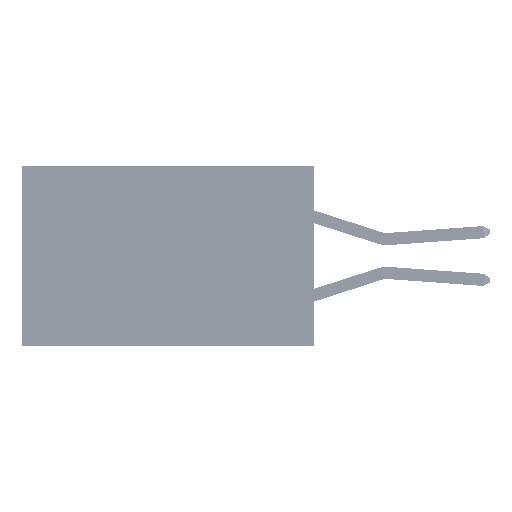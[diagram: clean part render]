
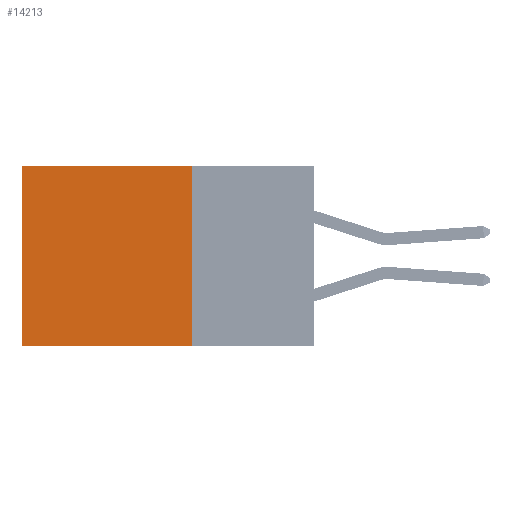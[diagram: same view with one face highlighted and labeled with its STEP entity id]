
A CAD part, left-side view. The second image highlights one B-rep face of the part: STEP entity #14213.
In plain terms, the highlighted planar face has unit normal (-1, 0, 0).
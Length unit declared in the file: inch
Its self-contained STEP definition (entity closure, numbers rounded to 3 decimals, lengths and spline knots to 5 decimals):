
#1226 = VERTEX_POINT ( 'NONE', #41984 ) ;
#1234 = CARTESIAN_POINT ( 'NONE',  ( 0.2875, 0.6, 0. ) ) ;
#1390 = DIRECTION ( 'NONE',  ( 0., 0., -1. ) ) ;
#2283 = EDGE_CURVE ( 'NONE', #33521, #27277, #3901, .T. ) ;
#3901 = LINE ( 'NONE', #34683, #35376 ) ;
#7206 = DIRECTION ( 'NONE',  ( 0., 0., -1. ) ) ;
#7825 = LINE ( 'NONE', #43653, #44966 ) ;
#9397 = DIRECTION ( 'NONE',  ( 0., 1., 0. ) ) ;
#10475 = ORIENTED_EDGE ( 'NONE', *, *, #2283, .F. ) ;
#13474 = VECTOR ( 'NONE', #43438, 39.37008 ) ;
#13929 = DIRECTION ( 'NONE',  ( 1., 0., 0. ) ) ;
#14095 = PLANE ( 'NONE',  #30364 ) ;
#14213 = ADVANCED_FACE ( 'NONE', ( #26748 ), #14095, .F. ) ;
#14412 = VERTEX_POINT ( 'NONE', #1234 ) ;
#14623 = DIRECTION ( 'NONE',  ( 0., 0., -1. ) ) ;
#15392 = VECTOR ( 'NONE', #9397, 39.37008 ) ;
#16209 = EDGE_LOOP ( 'NONE', ( #30724, #36020, #10475, #21837 ) ) ;
#17731 = CARTESIAN_POINT ( 'NONE',  ( 0.2875, 0.25, -0.37 ) ) ;
#20446 = CARTESIAN_POINT ( 'NONE',  ( 0.2875, 0.25, 0. ) ) ;
#21837 = ORIENTED_EDGE ( 'NONE', *, *, #45774, .T. ) ;
#22580 = CARTESIAN_POINT ( 'NONE',  ( 0.2875, 0.25, -0.37 ) ) ;
#23207 = LINE ( 'NONE', #17731, #13474 ) ;
#25975 = EDGE_CURVE ( 'NONE', #27277, #1226, #23207, .T. ) ;
#26748 = FACE_OUTER_BOUND ( 'NONE', #16209, .T. ) ;
#27277 = VERTEX_POINT ( 'NONE', #22580 ) ;
#30364 = AXIS2_PLACEMENT_3D ( 'NONE', #42995, #13929, #7206 ) ;
#30724 = ORIENTED_EDGE ( 'NONE', *, *, #47180, .T. ) ;
#33521 = VERTEX_POINT ( 'NONE', #46909 ) ;
#34683 = CARTESIAN_POINT ( 'NONE',  ( 0.2875, 0.25, 0. ) ) ;
#35376 = VECTOR ( 'NONE', #1390, 39.37008 ) ;
#36020 = ORIENTED_EDGE ( 'NONE', *, *, #25975, .F. ) ;
#37147 = LINE ( 'NONE', #20446, #15392 ) ;
#41984 = CARTESIAN_POINT ( 'NONE',  ( 0.2875, 0.6, -0.37 ) ) ;
#42995 = CARTESIAN_POINT ( 'NONE',  ( 0.2875, 0.25, 0. ) ) ;
#43438 = DIRECTION ( 'NONE',  ( 0., 1., 0. ) ) ;
#43653 = CARTESIAN_POINT ( 'NONE',  ( 0.2875, 0.6, 0. ) ) ;
#44966 = VECTOR ( 'NONE', #14623, 39.37008 ) ;
#45774 = EDGE_CURVE ( 'NONE', #33521, #14412, #37147, .T. ) ;
#46909 = CARTESIAN_POINT ( 'NONE',  ( 0.2875, 0.25, 0. ) ) ;
#47180 = EDGE_CURVE ( 'NONE', #14412, #1226, #7825, .T. ) ;
